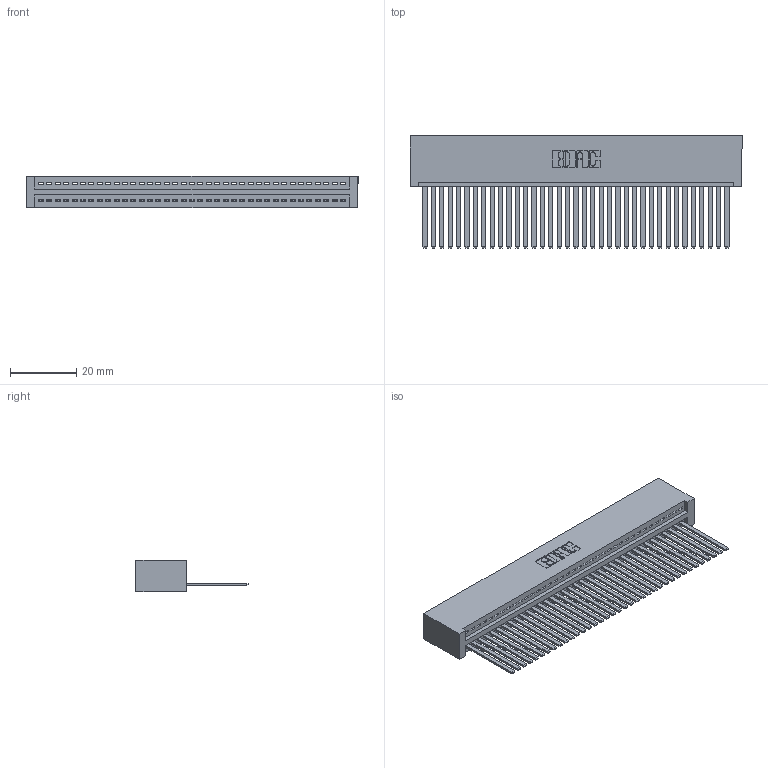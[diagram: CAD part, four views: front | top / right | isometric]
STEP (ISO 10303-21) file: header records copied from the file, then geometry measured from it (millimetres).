
FILE_DESCRIPTION (( 'STEP AP203' ), '1' );
FILE_NAME ('395-037-544-101.STEP', '2018-11-14T00:13:38', ( '' ), ( '' ), 'SwSTEP 2.0', 'SolidWorks 2016', '' );
FILE_SCHEMA (( 'CONFIG_CONTROL_DESIGN' ));
Length unit declared in the file: inch
Products named in the file (3): 345 Part_No Mounting Lugs; 345-292-001_345-293-144; 395-037-544-101
Assembly tree (38 placements, depth 2):
  395-037-544-101
    345 Part_No Mounting Lugs
    345-292-001_345-293-144  x37
Bounding box: 100.58 x 33.96 x 9.4 mm (x, y, z)
Volume: 10525.5 mm3; surface area: 15396 mm2
Topology: 38 solids, 38 shells, 2042 faces, 6163 edges, 4058 vertices
Faces by surface type: plane 1408, cylinder 634
Entity records: 28059 total; most frequent: CARTESIAN_POINT 4867, ORIENTED_EDGE 4838, DIRECTION 4249, EDGE_CURVE 2419, VECTOR 2151, LINE 2151, VERTEX_POINT 1610, AXIS2_PLACEMENT_3D 1049
